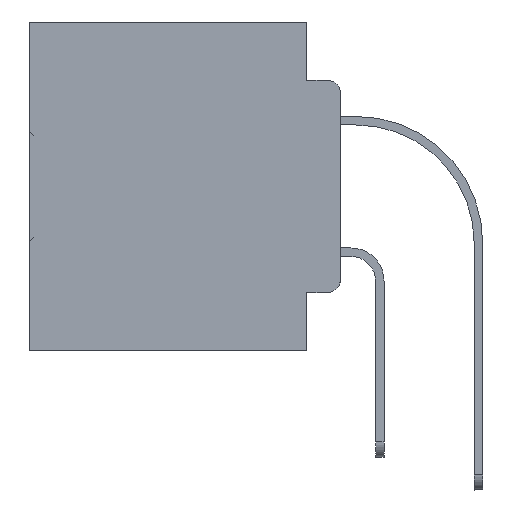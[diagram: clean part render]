
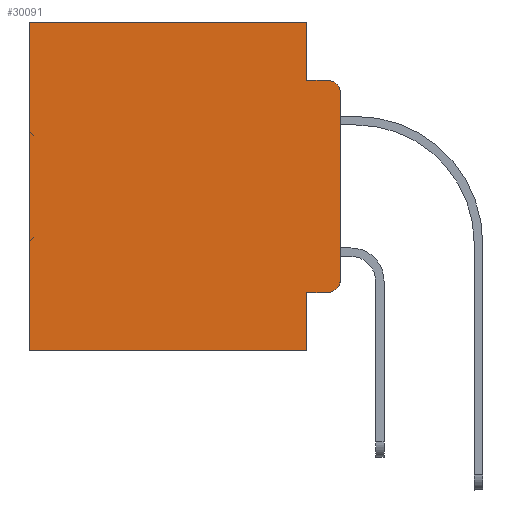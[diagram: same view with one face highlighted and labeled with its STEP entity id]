
A CAD part, left-side view. The second image highlights one B-rep face of the part: STEP entity #30091.
In plain terms, the highlighted planar face has unit normal (-1, 0, 0).
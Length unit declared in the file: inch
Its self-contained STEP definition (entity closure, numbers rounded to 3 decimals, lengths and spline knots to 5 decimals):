
#134 = VERTEX_POINT ( 'NONE', #16462 ) ;
#261 = CARTESIAN_POINT ( 'NONE',  ( 0.298, 0.051, -0.5 ) ) ;
#492 = CARTESIAN_POINT ( 'NONE',  ( 0.298, 0.051, 0. ) ) ;
#787 = EDGE_CURVE ( 'NONE', #134, #20998, #8399, .T. ) ;
#1397 = CARTESIAN_POINT ( 'NONE',  ( 0.298, 0.02, -0.1085 ) ) ;
#1414 = DIRECTION ( 'NONE',  ( 0., 0., -1. ) ) ;
#1555 = VERTEX_POINT ( 'NONE', #261 ) ;
#1792 = CARTESIAN_POINT ( 'NONE',  ( 0.298, 0.02, -0.3915 ) ) ;
#2290 = CARTESIAN_POINT ( 'NONE',  ( 0.298, 0.02, -0.0885 ) ) ;
#2301 = VERTEX_POINT ( 'NONE', #23982 ) ;
#2848 = VECTOR ( 'NONE', #33163, 39.37008 ) ;
#4919 = VECTOR ( 'NONE', #6769, 39.37008 ) ;
#5228 = FACE_OUTER_BOUND ( 'NONE', #15112, .T. ) ;
#6315 = LINE ( 'NONE', #17299, #15058 ) ;
#6769 = DIRECTION ( 'NONE',  ( 0., 0., -1. ) ) ;
#6842 = CARTESIAN_POINT ( 'NONE',  ( 0.298, 0.051, 0. ) ) ;
#7924 = DIRECTION ( 'NONE',  ( 0., -1., 0. ) ) ;
#8399 = LINE ( 'NONE', #20083, #13083 ) ;
#8549 = PLANE ( 'NONE',  #37516 ) ;
#8596 = DIRECTION ( 'NONE',  ( 0., -1., 0. ) ) ;
#9427 = CARTESIAN_POINT ( 'NONE',  ( 0.298, 0., -0.3915 ) ) ;
#9841 = CARTESIAN_POINT ( 'NONE',  ( 0.298, 0., -0.1085 ) ) ;
#10707 = VERTEX_POINT ( 'NONE', #21521 ) ;
#12494 = CARTESIAN_POINT ( 'NONE',  ( 0.298, 0.473, 0. ) ) ;
#12511 = EDGE_CURVE ( 'NONE', #24950, #37208, #22376, .T. ) ;
#13083 = VECTOR ( 'NONE', #8596, 39.37008 ) ;
#13089 = DIRECTION ( 'NONE',  ( 0., 0., -1. ) ) ;
#13127 = VECTOR ( 'NONE', #36329, 39.37008 ) ;
#13284 = DIRECTION ( 'NONE',  ( -1., 0., 0. ) ) ;
#13396 = ORIENTED_EDGE ( 'NONE', *, *, #21501, .F. ) ;
#14321 = ORIENTED_EDGE ( 'NONE', *, *, #19090, .T. ) ;
#14415 = CARTESIAN_POINT ( 'NONE',  ( 0.298, 0.02, -0.4115 ) ) ;
#14535 = ORIENTED_EDGE ( 'NONE', *, *, #787, .T. ) ;
#14808 = VERTEX_POINT ( 'NONE', #28070 ) ;
#15048 = EDGE_CURVE ( 'NONE', #36619, #2301, #18428, .T. ) ;
#15058 = VECTOR ( 'NONE', #37582, 39.37008 ) ;
#15112 = EDGE_LOOP ( 'NONE', ( #15635, #36340, #20095, #17717, #17580, #23364, #13396, #27513, #14535, #14321 ) ) ;
#15635 = ORIENTED_EDGE ( 'NONE', *, *, #27581, .F. ) ;
#16175 = CIRCLE ( 'NONE', #34204, 0.02 ) ;
#16462 = CARTESIAN_POINT ( 'NONE',  ( 0.298, 0.051, -0.4115 ) ) ;
#16606 = EDGE_CURVE ( 'NONE', #2301, #37208, #34641, .T. ) ;
#17101 = CARTESIAN_POINT ( 'NONE',  ( 0.298, 0.051, -0.0885 ) ) ;
#17299 = CARTESIAN_POINT ( 'NONE',  ( 0.298, 0., -0.5 ) ) ;
#17580 = ORIENTED_EDGE ( 'NONE', *, *, #20275, .T. ) ;
#17717 = ORIENTED_EDGE ( 'NONE', *, *, #15048, .F. ) ;
#18428 = LINE ( 'NONE', #492, #24375 ) ;
#18964 = CARTESIAN_POINT ( 'NONE',  ( 0.298, 0., 0. ) ) ;
#19090 = EDGE_CURVE ( 'NONE', #20998, #21613, #16175, .T. ) ;
#19400 = LINE ( 'NONE', #35001, #31596 ) ;
#19889 = AXIS2_PLACEMENT_3D ( 'NONE', #1397, #13284, #13089 ) ;
#20083 = CARTESIAN_POINT ( 'NONE',  ( 0.298, 0.051, -0.4115 ) ) ;
#20095 = ORIENTED_EDGE ( 'NONE', *, *, #16606, .F. ) ;
#20158 = DIRECTION ( 'NONE',  ( 0., 0., -1. ) ) ;
#20275 = EDGE_CURVE ( 'NONE', #36619, #10707, #24423, .T. ) ;
#20998 = VERTEX_POINT ( 'NONE', #14415 ) ;
#21501 = EDGE_CURVE ( 'NONE', #1555, #14808, #6315, .T. ) ;
#21521 = CARTESIAN_POINT ( 'NONE',  ( 0.298, 0.473, 0. ) ) ;
#21613 = VERTEX_POINT ( 'NONE', #9427 ) ;
#22376 = CIRCLE ( 'NONE', #19889, 0.02 ) ;
#23099 = EDGE_CURVE ( 'NONE', #134, #1555, #27631, .T. ) ;
#23364 = ORIENTED_EDGE ( 'NONE', *, *, #35119, .T. ) ;
#23726 = DIRECTION ( 'NONE',  ( 0., 0., -1. ) ) ;
#23982 = CARTESIAN_POINT ( 'NONE',  ( 0.298, 0.051, -0.0885 ) ) ;
#24375 = VECTOR ( 'NONE', #27590, 39.37008 ) ;
#24423 = LINE ( 'NONE', #18964, #13127 ) ;
#24950 = VERTEX_POINT ( 'NONE', #9841 ) ;
#27513 = ORIENTED_EDGE ( 'NONE', *, *, #23099, .F. ) ;
#27581 = EDGE_CURVE ( 'NONE', #24950, #21613, #19400, .T. ) ;
#27590 = DIRECTION ( 'NONE',  ( 0., 0., -1. ) ) ;
#27631 = LINE ( 'NONE', #31135, #4919 ) ;
#28070 = CARTESIAN_POINT ( 'NONE',  ( 0.298, 0.473, -0.5 ) ) ;
#29470 = LINE ( 'NONE', #12494, #2848 ) ;
#30091 = ADVANCED_FACE ( 'NONE', ( #5228 ), #8549, .F. ) ;
#31135 = CARTESIAN_POINT ( 'NONE',  ( 0.298, 0.051, 0. ) ) ;
#31596 = VECTOR ( 'NONE', #20158, 39.37008 ) ;
#32518 = VECTOR ( 'NONE', #7924, 39.37008 ) ;
#33163 = DIRECTION ( 'NONE',  ( 0., 0., -1. ) ) ;
#33978 = DIRECTION ( 'NONE',  ( -1., 0., 0. ) ) ;
#34204 = AXIS2_PLACEMENT_3D ( 'NONE', #1792, #33978, #1414 ) ;
#34641 = LINE ( 'NONE', #17101, #32518 ) ;
#34859 = CARTESIAN_POINT ( 'NONE',  ( 0.298, 0., 0. ) ) ;
#35001 = CARTESIAN_POINT ( 'NONE',  ( 0.298, 0., 0. ) ) ;
#35119 = EDGE_CURVE ( 'NONE', #10707, #14808, #29470, .T. ) ;
#36329 = DIRECTION ( 'NONE',  ( 0., 1., 0. ) ) ;
#36340 = ORIENTED_EDGE ( 'NONE', *, *, #12511, .T. ) ;
#36619 = VERTEX_POINT ( 'NONE', #6842 ) ;
#37208 = VERTEX_POINT ( 'NONE', #2290 ) ;
#37516 = AXIS2_PLACEMENT_3D ( 'NONE', #34859, #37800, #23726 ) ;
#37582 = DIRECTION ( 'NONE',  ( 0., 1., 0. ) ) ;
#37800 = DIRECTION ( 'NONE',  ( 1., 0., 0. ) ) ;
